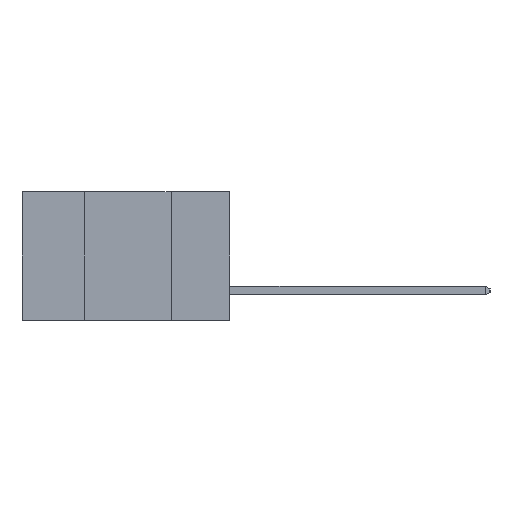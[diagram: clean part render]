
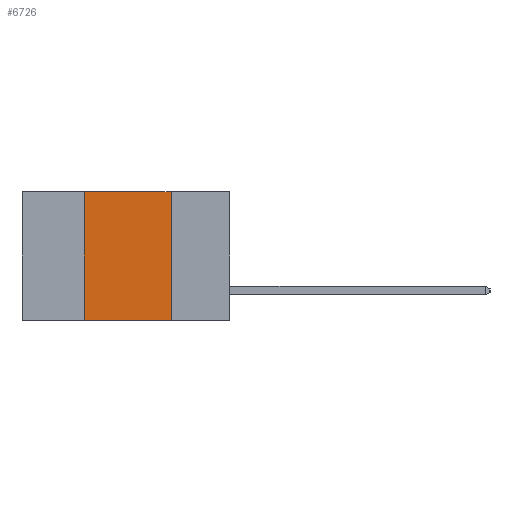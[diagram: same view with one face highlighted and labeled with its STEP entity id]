
A CAD part, left-side view. The second image highlights one B-rep face of the part: STEP entity #6726.
In plain terms, the highlighted planar face has unit normal (-1, 0, 0).
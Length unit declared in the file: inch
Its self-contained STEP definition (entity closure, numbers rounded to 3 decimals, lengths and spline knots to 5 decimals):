
#274 = EDGE_CURVE ( 'NONE', #1871, #1564, #3845, .T. ) ;
#1010 = DIRECTION ( 'NONE',  ( 0., 0., -1. ) ) ;
#1026 = DIRECTION ( 'NONE',  ( 1., 0., 0. ) ) ;
#1194 = PLANE ( 'NONE',  #10941 ) ;
#1453 = CARTESIAN_POINT ( 'NONE',  ( 0., 0.6, 0. ) ) ;
#1564 = VERTEX_POINT ( 'NONE', #7559 ) ;
#1871 = VERTEX_POINT ( 'NONE', #2263 ) ;
#2263 = CARTESIAN_POINT ( 'NONE',  ( 0., 0.42, -0.37 ) ) ;
#3041 = CARTESIAN_POINT ( 'NONE',  ( 0., 0.17, -0.37 ) ) ;
#3184 = DIRECTION ( 'NONE',  ( 0., 0., -1. ) ) ;
#3720 = ORIENTED_EDGE ( 'NONE', *, *, #4303, .T. ) ;
#3845 = LINE ( 'NONE', #7354, #4129 ) ;
#4129 = VECTOR ( 'NONE', #7707, 39.37008 ) ;
#4303 = EDGE_CURVE ( 'NONE', #1871, #9506, #7235, .T. ) ;
#5277 = VERTEX_POINT ( 'NONE', #7994 ) ;
#5719 = EDGE_CURVE ( 'NONE', #5277, #9506, #10616, .T. ) ;
#6081 = VECTOR ( 'NONE', #3184, 39.37008 ) ;
#6493 = EDGE_LOOP ( 'NONE', ( #6868, #7046, #7506, #3720 ) ) ;
#6726 = ADVANCED_FACE ( 'NONE', ( #8770 ), #1194, .F. ) ;
#6868 = ORIENTED_EDGE ( 'NONE', *, *, #5719, .F. ) ;
#7046 = ORIENTED_EDGE ( 'NONE', *, *, #9225, .F. ) ;
#7051 = LINE ( 'NONE', #8402, #11226 ) ;
#7235 = LINE ( 'NONE', #10272, #11388 ) ;
#7354 = CARTESIAN_POINT ( 'NONE',  ( 0., 0.42, -0.37 ) ) ;
#7506 = ORIENTED_EDGE ( 'NONE', *, *, #274, .F. ) ;
#7559 = CARTESIAN_POINT ( 'NONE',  ( 0., 0.42, 0. ) ) ;
#7707 = DIRECTION ( 'NONE',  ( 0., 0., 1. ) ) ;
#7994 = CARTESIAN_POINT ( 'NONE',  ( 0., 0.17, 0. ) ) ;
#8168 = CARTESIAN_POINT ( 'NONE',  ( 0., 0.17, -0.37 ) ) ;
#8402 = CARTESIAN_POINT ( 'NONE',  ( 0., 0.6, 0. ) ) ;
#8770 = FACE_OUTER_BOUND ( 'NONE', #6493, .T. ) ;
#8780 = DIRECTION ( 'NONE',  ( 0., -1., 0. ) ) ;
#9225 = EDGE_CURVE ( 'NONE', #1564, #5277, #7051, .T. ) ;
#9506 = VERTEX_POINT ( 'NONE', #8168 ) ;
#9983 = DIRECTION ( 'NONE',  ( 0., -1., 0. ) ) ;
#10272 = CARTESIAN_POINT ( 'NONE',  ( 0., 0.6, -0.37 ) ) ;
#10616 = LINE ( 'NONE', #3041, #6081 ) ;
#10941 = AXIS2_PLACEMENT_3D ( 'NONE', #1453, #1026, #1010 ) ;
#11226 = VECTOR ( 'NONE', #8780, 39.37008 ) ;
#11388 = VECTOR ( 'NONE', #9983, 39.37008 ) ;
